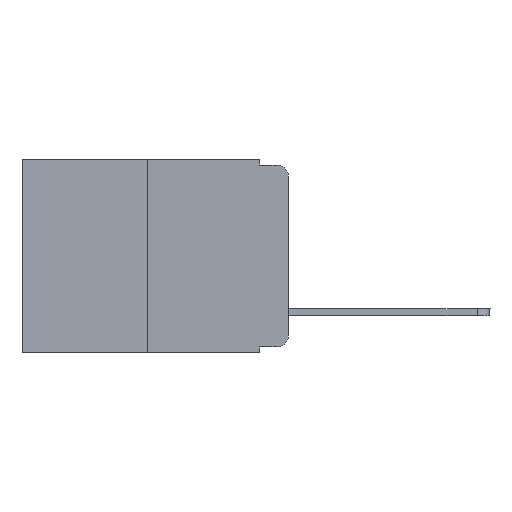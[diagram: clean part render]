
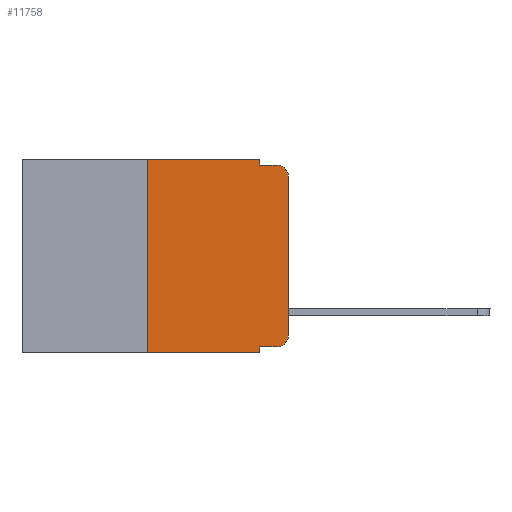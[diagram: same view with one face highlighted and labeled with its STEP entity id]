
A CAD part, left-side view. The second image highlights one B-rep face of the part: STEP entity #11758.
In plain terms, the highlighted planar face has unit normal (-1, 0, 0).
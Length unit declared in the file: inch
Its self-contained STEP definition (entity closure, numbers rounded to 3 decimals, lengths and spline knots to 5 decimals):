
#69 = CARTESIAN_POINT ( 'NONE',  ( 0., 0.051, 0. ) ) ;
#98 = EDGE_CURVE ( 'NONE', #9993, #5199, #14650, .T. ) ;
#747 = PLANE ( 'NONE',  #13086 ) ;
#1250 = CARTESIAN_POINT ( 'NONE',  ( 0., 0.051, -0.01 ) ) ;
#1288 = VECTOR ( 'NONE', #9719, 39.37008 ) ;
#1750 = DIRECTION ( 'NONE',  ( 0., -1., 0. ) ) ;
#1998 = VERTEX_POINT ( 'NONE', #6544 ) ;
#2095 = CARTESIAN_POINT ( 'NONE',  ( 0., 0., 0. ) ) ;
#2692 = CARTESIAN_POINT ( 'NONE',  ( 0., 0.473, 0. ) ) ;
#2832 = DIRECTION ( 'NONE',  ( 0., 0., 1. ) ) ;
#2834 = CARTESIAN_POINT ( 'NONE',  ( 0., 0.02, -0.333 ) ) ;
#3299 = ORIENTED_EDGE ( 'NONE', *, *, #16718, .T. ) ;
#3550 = VERTEX_POINT ( 'NONE', #12854 ) ;
#3573 = ORIENTED_EDGE ( 'NONE', *, *, #15467, .T. ) ;
#3688 = EDGE_CURVE ( 'NONE', #3550, #9993, #9508, .T. ) ;
#3836 = DIRECTION ( 'NONE',  ( -1., 0., 0. ) ) ;
#4133 = CARTESIAN_POINT ( 'NONE',  ( 0., 0.051, 0. ) ) ;
#4224 = DIRECTION ( 'NONE',  ( 0., -1., 0. ) ) ;
#4507 = DIRECTION ( 'NONE',  ( 1., 0., 0. ) ) ;
#4978 = CIRCLE ( 'NONE', #17029, 0.02 ) ;
#5074 = EDGE_LOOP ( 'NONE', ( #15301, #3299, #15933, #11091, #8132, #9699, #6165, #16254, #8176, #3573 ) ) ;
#5199 = VERTEX_POINT ( 'NONE', #4133 ) ;
#5312 = DIRECTION ( 'NONE',  ( 0., 0., -1. ) ) ;
#5445 = EDGE_CURVE ( 'NONE', #8350, #16410, #12890, .T. ) ;
#6165 = ORIENTED_EDGE ( 'NONE', *, *, #10711, .T. ) ;
#6544 = CARTESIAN_POINT ( 'NONE',  ( 0., 0.051, -0.333 ) ) ;
#6984 = LINE ( 'NONE', #69, #1288 ) ;
#7247 = CARTESIAN_POINT ( 'NONE',  ( 0., 0.25, 0. ) ) ;
#8010 = VECTOR ( 'NONE', #4224, 39.37008 ) ;
#8132 = ORIENTED_EDGE ( 'NONE', *, *, #98, .F. ) ;
#8171 = CARTESIAN_POINT ( 'NONE',  ( 0., 0., -0.313 ) ) ;
#8176 = ORIENTED_EDGE ( 'NONE', *, *, #10690, .T. ) ;
#8350 = VERTEX_POINT ( 'NONE', #8171 ) ;
#8423 = AXIS2_PLACEMENT_3D ( 'NONE', #17340, #16118, #5312 ) ;
#8601 = VECTOR ( 'NONE', #2832, 39.37008 ) ;
#9151 = CARTESIAN_POINT ( 'NONE',  ( 0., 0.051, -0.01 ) ) ;
#9481 = CARTESIAN_POINT ( 'NONE',  ( 0., 0.02, -0.01 ) ) ;
#9508 = LINE ( 'NONE', #14874, #8601 ) ;
#9546 = CARTESIAN_POINT ( 'NONE',  ( 0., 0.051, 0. ) ) ;
#9674 = VECTOR ( 'NONE', #11959, 39.37008 ) ;
#9699 = ORIENTED_EDGE ( 'NONE', *, *, #3688, .F. ) ;
#9719 = DIRECTION ( 'NONE',  ( 0., 0., -1. ) ) ;
#9749 = LINE ( 'NONE', #13521, #11662 ) ;
#9836 = CARTESIAN_POINT ( 'NONE',  ( 0., 0.473, -0.343 ) ) ;
#9993 = VERTEX_POINT ( 'NONE', #7247 ) ;
#10136 = CARTESIAN_POINT ( 'NONE',  ( 0., 0.473, 0. ) ) ;
#10325 = VERTEX_POINT ( 'NONE', #11271 ) ;
#10451 = VERTEX_POINT ( 'NONE', #9151 ) ;
#10512 = EDGE_CURVE ( 'NONE', #10451, #13484, #11875, .T. ) ;
#10690 = EDGE_CURVE ( 'NONE', #1998, #11899, #9749, .T. ) ;
#10711 = EDGE_CURVE ( 'NONE', #3550, #10325, #16506, .T. ) ;
#11043 = LINE ( 'NONE', #9546, #16707 ) ;
#11079 = EDGE_CURVE ( 'NONE', #5199, #10451, #6984, .T. ) ;
#11091 = ORIENTED_EDGE ( 'NONE', *, *, #11079, .F. ) ;
#11193 = FACE_OUTER_BOUND ( 'NONE', #5074, .T. ) ;
#11271 = CARTESIAN_POINT ( 'NONE',  ( 0., 0.051, -0.343 ) ) ;
#11662 = VECTOR ( 'NONE', #1750, 39.37008 ) ;
#11758 = ADVANCED_FACE ( 'NONE', ( #11193 ), #747, .F. ) ;
#11875 = LINE ( 'NONE', #1250, #9674 ) ;
#11899 = VERTEX_POINT ( 'NONE', #2834 ) ;
#11959 = DIRECTION ( 'NONE',  ( 0., -1., 0. ) ) ;
#12854 = CARTESIAN_POINT ( 'NONE',  ( 0., 0.25, -0.343 ) ) ;
#12890 = LINE ( 'NONE', #2095, #14916 ) ;
#13086 = AXIS2_PLACEMENT_3D ( 'NONE', #10136, #4507, #15503 ) ;
#13406 = DIRECTION ( 'NONE',  ( 0., -1., 0. ) ) ;
#13484 = VERTEX_POINT ( 'NONE', #9481 ) ;
#13521 = CARTESIAN_POINT ( 'NONE',  ( 0., 0.051, -0.333 ) ) ;
#14559 = DIRECTION ( 'NONE',  ( 0., 0., -1. ) ) ;
#14650 = LINE ( 'NONE', #2692, #16952 ) ;
#14874 = CARTESIAN_POINT ( 'NONE',  ( 0., 0.25, 0. ) ) ;
#14916 = VECTOR ( 'NONE', #17105, 39.37008 ) ;
#15077 = DIRECTION ( 'NONE',  ( 0., 0., -1. ) ) ;
#15301 = ORIENTED_EDGE ( 'NONE', *, *, #5445, .T. ) ;
#15467 = EDGE_CURVE ( 'NONE', #11899, #8350, #15748, .T. ) ;
#15503 = DIRECTION ( 'NONE',  ( 0., 0., -1. ) ) ;
#15748 = CIRCLE ( 'NONE', #8423, 0.02 ) ;
#15879 = CARTESIAN_POINT ( 'NONE',  ( 0., 0.02, -0.03 ) ) ;
#15933 = ORIENTED_EDGE ( 'NONE', *, *, #10512, .F. ) ;
#16118 = DIRECTION ( 'NONE',  ( -1., 0., 0. ) ) ;
#16142 = CARTESIAN_POINT ( 'NONE',  ( 0., 0., -0.03 ) ) ;
#16254 = ORIENTED_EDGE ( 'NONE', *, *, #16376, .F. ) ;
#16376 = EDGE_CURVE ( 'NONE', #1998, #10325, #11043, .T. ) ;
#16410 = VERTEX_POINT ( 'NONE', #16142 ) ;
#16506 = LINE ( 'NONE', #9836, #8010 ) ;
#16707 = VECTOR ( 'NONE', #15077, 39.37008 ) ;
#16718 = EDGE_CURVE ( 'NONE', #16410, #13484, #4978, .T. ) ;
#16952 = VECTOR ( 'NONE', #13406, 39.37008 ) ;
#17029 = AXIS2_PLACEMENT_3D ( 'NONE', #15879, #3836, #14559 ) ;
#17105 = DIRECTION ( 'NONE',  ( 0., 0., 1. ) ) ;
#17340 = CARTESIAN_POINT ( 'NONE',  ( 0., 0.02, -0.313 ) ) ;
